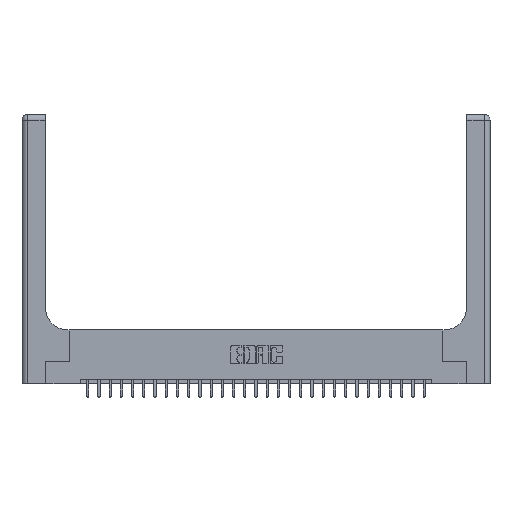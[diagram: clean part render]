
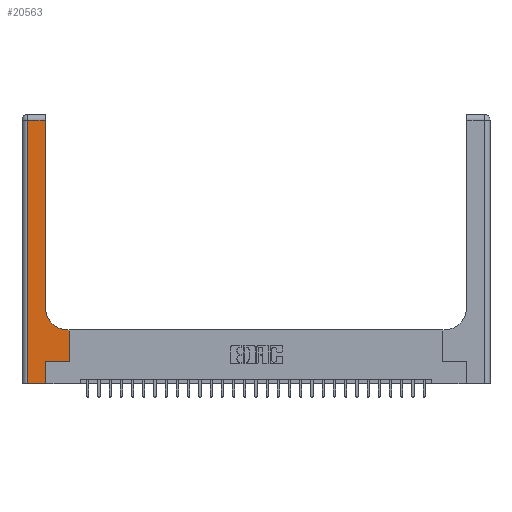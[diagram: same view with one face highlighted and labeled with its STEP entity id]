
A CAD part, top view. The second image highlights one B-rep face of the part: STEP entity #20563.
In plain terms, the highlighted planar face has unit normal (0, 0, 1).
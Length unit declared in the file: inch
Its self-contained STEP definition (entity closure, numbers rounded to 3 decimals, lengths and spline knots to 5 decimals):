
#28 = DIRECTION ( 'NONE',  ( 0., 0., -1. ) ) ;
#1545 = CARTESIAN_POINT ( 'NONE',  ( 0.265, 0., 0.37 ) ) ;
#1632 = EDGE_CURVE ( 'NONE', #26071, #19959, #17926, .T. ) ;
#1921 = DIRECTION ( 'NONE',  ( -1., 0., 0. ) ) ;
#2388 = CARTESIAN_POINT ( 'NONE',  ( 0.265, 0.25, 0.37 ) ) ;
#2526 = EDGE_CURVE ( 'NONE', #10946, #11544, #14640, .T. ) ;
#2911 = LINE ( 'NONE', #25872, #26654 ) ;
#4128 = CARTESIAN_POINT ( 'NONE',  ( 0., 3., 0.37 ) ) ;
#4344 = ORIENTED_EDGE ( 'NONE', *, *, #2526, .T. ) ;
#4798 = CARTESIAN_POINT ( 'NONE',  ( 0.26, 3., 0.37 ) ) ;
#4820 = CARTESIAN_POINT ( 'NONE',  ( 0., 2.94, 0.37 ) ) ;
#4849 = VECTOR ( 'NONE', #14938, 39.37008 ) ;
#4878 = DIRECTION ( 'NONE',  ( 0., -1., 0. ) ) ;
#5029 = ORIENTED_EDGE ( 'NONE', *, *, #1632, .T. ) ;
#5089 = AXIS2_PLACEMENT_3D ( 'NONE', #4128, #28, #1921 ) ;
#5249 = DIRECTION ( 'NONE',  ( -1., 0., 0. ) ) ;
#5555 = CARTESIAN_POINT ( 'NONE',  ( 0.528, 0.25, 0.37 ) ) ;
#6075 = LINE ( 'NONE', #21887, #24588 ) ;
#6103 = EDGE_CURVE ( 'NONE', #25010, #12571, #12363, .T. ) ;
#6908 = CARTESIAN_POINT ( 'NONE',  ( 0.265, 0., 0.37 ) ) ;
#7083 = AXIS2_PLACEMENT_3D ( 'NONE', #11089, #13518, #21483 ) ;
#7556 = EDGE_CURVE ( 'NONE', #19525, #25010, #6075, .T. ) ;
#7833 = CARTESIAN_POINT ( 'NONE',  ( 0.26, 0.85, 0.37 ) ) ;
#7845 = EDGE_CURVE ( 'NONE', #19382, #19525, #10969, .T. ) ;
#8024 = ORIENTED_EDGE ( 'NONE', *, *, #13666, .T. ) ;
#9683 = DIRECTION ( 'NONE',  ( 0., 1., 0. ) ) ;
#9971 = CARTESIAN_POINT ( 'NONE',  ( 0.06, 0., 0.37 ) ) ;
#10244 = ORIENTED_EDGE ( 'NONE', *, *, #7845, .T. ) ;
#10440 = CARTESIAN_POINT ( 'NONE',  ( 0.51, 0.6, 0.37 ) ) ;
#10563 = CARTESIAN_POINT ( 'NONE',  ( 0.528, 0.6, 0.37 ) ) ;
#10946 = VERTEX_POINT ( 'NONE', #10440 ) ;
#10969 = LINE ( 'NONE', #17248, #23904 ) ;
#11089 = CARTESIAN_POINT ( 'NONE',  ( 0.51, 0.85, 0.37 ) ) ;
#11394 = LINE ( 'NONE', #2388, #4849 ) ;
#11544 = VERTEX_POINT ( 'NONE', #7833 ) ;
#12363 = LINE ( 'NONE', #1545, #14288 ) ;
#12571 = VERTEX_POINT ( 'NONE', #13442 ) ;
#13002 = LINE ( 'NONE', #4798, #16209 ) ;
#13442 = CARTESIAN_POINT ( 'NONE',  ( 0.265, 0.25, 0.37 ) ) ;
#13518 = DIRECTION ( 'NONE',  ( 0., 0., -1. ) ) ;
#13575 = DIRECTION ( 'NONE',  ( 1., 0., 0. ) ) ;
#13666 = EDGE_CURVE ( 'NONE', #11544, #14226, #13002, .T. ) ;
#13700 = CARTESIAN_POINT ( 'NONE',  ( 0.06, 2.94, 0.37 ) ) ;
#14226 = VERTEX_POINT ( 'NONE', #19457 ) ;
#14288 = VECTOR ( 'NONE', #9683, 39.37008 ) ;
#14640 = CIRCLE ( 'NONE', #7083, 0.25 ) ;
#14666 = LINE ( 'NONE', #4820, #22131 ) ;
#14938 = DIRECTION ( 'NONE',  ( 1., 0., 0. ) ) ;
#15731 = EDGE_LOOP ( 'NONE', ( #8024, #20892, #10244, #22399, #26828, #24855, #5029, #20295, #4344 ) ) ;
#16209 = VECTOR ( 'NONE', #19313, 39.37008 ) ;
#17248 = CARTESIAN_POINT ( 'NONE',  ( 0.06, 3., 0.37 ) ) ;
#17926 = LINE ( 'NONE', #5555, #22799 ) ;
#18736 = CARTESIAN_POINT ( 'NONE',  ( 0.528, 0.25, 0.37 ) ) ;
#19313 = DIRECTION ( 'NONE',  ( 0., 1., 0. ) ) ;
#19382 = VERTEX_POINT ( 'NONE', #13700 ) ;
#19457 = CARTESIAN_POINT ( 'NONE',  ( 0.26, 2.94, 0.37 ) ) ;
#19525 = VERTEX_POINT ( 'NONE', #9971 ) ;
#19959 = VERTEX_POINT ( 'NONE', #10563 ) ;
#20295 = ORIENTED_EDGE ( 'NONE', *, *, #25141, .T. ) ;
#20563 = ADVANCED_FACE ( 'NONE', ( #25038 ), #26759, .F. ) ;
#20892 = ORIENTED_EDGE ( 'NONE', *, *, #24377, .T. ) ;
#21267 = DIRECTION ( 'NONE',  ( -1., 0., 0. ) ) ;
#21483 = DIRECTION ( 'NONE',  ( 1., 0., 0. ) ) ;
#21886 = DIRECTION ( 'NONE',  ( 0., 1., 0. ) ) ;
#21887 = CARTESIAN_POINT ( 'NONE',  ( 0., 0., 0.37 ) ) ;
#22131 = VECTOR ( 'NONE', #21267, 39.37008 ) ;
#22399 = ORIENTED_EDGE ( 'NONE', *, *, #7556, .T. ) ;
#22799 = VECTOR ( 'NONE', #21886, 39.37008 ) ;
#23904 = VECTOR ( 'NONE', #4878, 39.37008 ) ;
#24377 = EDGE_CURVE ( 'NONE', #14226, #19382, #14666, .T. ) ;
#24588 = VECTOR ( 'NONE', #13575, 39.37008 ) ;
#24855 = ORIENTED_EDGE ( 'NONE', *, *, #25589, .T. ) ;
#25010 = VERTEX_POINT ( 'NONE', #6908 ) ;
#25038 = FACE_OUTER_BOUND ( 'NONE', #15731, .T. ) ;
#25141 = EDGE_CURVE ( 'NONE', #19959, #10946, #2911, .T. ) ;
#25589 = EDGE_CURVE ( 'NONE', #12571, #26071, #11394, .T. ) ;
#25872 = CARTESIAN_POINT ( 'NONE',  ( 0.26, 0.6, 0.37 ) ) ;
#26071 = VERTEX_POINT ( 'NONE', #18736 ) ;
#26654 = VECTOR ( 'NONE', #5249, 39.37008 ) ;
#26759 = PLANE ( 'NONE',  #5089 ) ;
#26828 = ORIENTED_EDGE ( 'NONE', *, *, #6103, .T. ) ;
